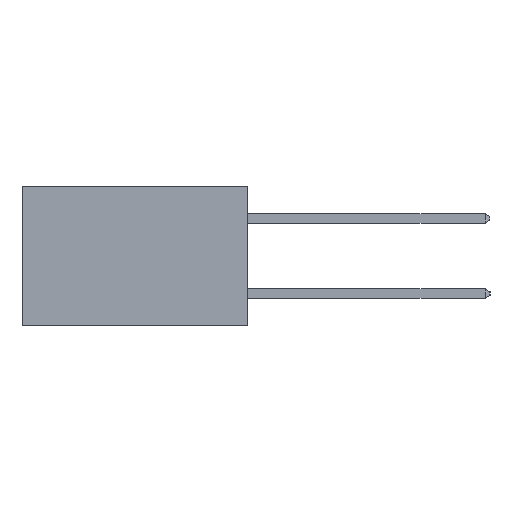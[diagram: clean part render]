
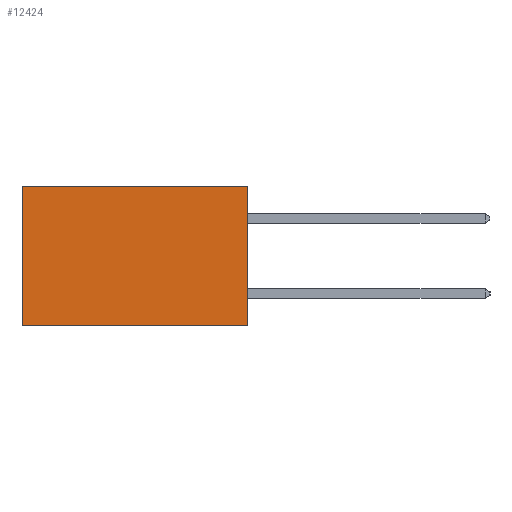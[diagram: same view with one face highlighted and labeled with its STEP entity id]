
A CAD part, left-side view. The second image highlights one B-rep face of the part: STEP entity #12424.
In plain terms, the highlighted planar face has unit normal (-1, 0, 0).
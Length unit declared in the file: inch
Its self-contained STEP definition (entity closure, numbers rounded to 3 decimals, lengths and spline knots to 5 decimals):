
#755 = DIRECTION ( 'NONE',  ( 0., 0., -1. ) ) ;
#1674 = VECTOR ( 'NONE', #25124, 39.37008 ) ;
#1909 = EDGE_CURVE ( 'NONE', #13738, #2033, #2335, .T. ) ;
#2033 = VERTEX_POINT ( 'NONE', #6042 ) ;
#2209 = ORIENTED_EDGE ( 'NONE', *, *, #14868, .T. ) ;
#2335 = LINE ( 'NONE', #8865, #1674 ) ;
#2985 = CARTESIAN_POINT ( 'NONE',  ( 0.2615, 0.6, 0. ) ) ;
#5100 = ORIENTED_EDGE ( 'NONE', *, *, #13733, .T. ) ;
#6042 = CARTESIAN_POINT ( 'NONE',  ( 0.2615, 0.6, -0.37 ) ) ;
#6348 = LINE ( 'NONE', #9958, #16392 ) ;
#7196 = LINE ( 'NONE', #22123, #22436 ) ;
#7659 = AXIS2_PLACEMENT_3D ( 'NONE', #10822, #12839, #755 ) ;
#8233 = DIRECTION ( 'NONE',  ( 0., 0., -1. ) ) ;
#8865 = CARTESIAN_POINT ( 'NONE',  ( 0.2615, 0., -0.37 ) ) ;
#9744 = ORIENTED_EDGE ( 'NONE', *, *, #18990, .F. ) ;
#9958 = CARTESIAN_POINT ( 'NONE',  ( 0.2615, 0., -0.37 ) ) ;
#10822 = CARTESIAN_POINT ( 'NONE',  ( 0.2615, 0., -0.37 ) ) ;
#10867 = VERTEX_POINT ( 'NONE', #15585 ) ;
#10887 = EDGE_LOOP ( 'NONE', ( #2209, #14854, #9744, #5100 ) ) ;
#12008 = DIRECTION ( 'NONE',  ( 0., 0., -1. ) ) ;
#12424 = ADVANCED_FACE ( 'NONE', ( #16438 ), #22655, .F. ) ;
#12771 = CARTESIAN_POINT ( 'NONE',  ( 0.2615, 0., 0. ) ) ;
#12839 = DIRECTION ( 'NONE',  ( 1., 0., 0. ) ) ;
#13733 = EDGE_CURVE ( 'NONE', #10867, #20086, #22199, .T. ) ;
#13738 = VERTEX_POINT ( 'NONE', #18652 ) ;
#14854 = ORIENTED_EDGE ( 'NONE', *, *, #1909, .F. ) ;
#14868 = EDGE_CURVE ( 'NONE', #20086, #2033, #7196, .T. ) ;
#15585 = CARTESIAN_POINT ( 'NONE',  ( 0.2615, 0., 0. ) ) ;
#16392 = VECTOR ( 'NONE', #12008, 39.37008 ) ;
#16438 = FACE_OUTER_BOUND ( 'NONE', #10887, .T. ) ;
#16966 = VECTOR ( 'NONE', #24530, 39.37008 ) ;
#18652 = CARTESIAN_POINT ( 'NONE',  ( 0.2615, 0., -0.37 ) ) ;
#18990 = EDGE_CURVE ( 'NONE', #10867, #13738, #6348, .T. ) ;
#20086 = VERTEX_POINT ( 'NONE', #2985 ) ;
#22123 = CARTESIAN_POINT ( 'NONE',  ( 0.2615, 0.6, -0.37 ) ) ;
#22199 = LINE ( 'NONE', #12771, #16966 ) ;
#22436 = VECTOR ( 'NONE', #8233, 39.37008 ) ;
#22655 = PLANE ( 'NONE',  #7659 ) ;
#24530 = DIRECTION ( 'NONE',  ( 0., 1., 0. ) ) ;
#25124 = DIRECTION ( 'NONE',  ( 0., 1., 0. ) ) ;
